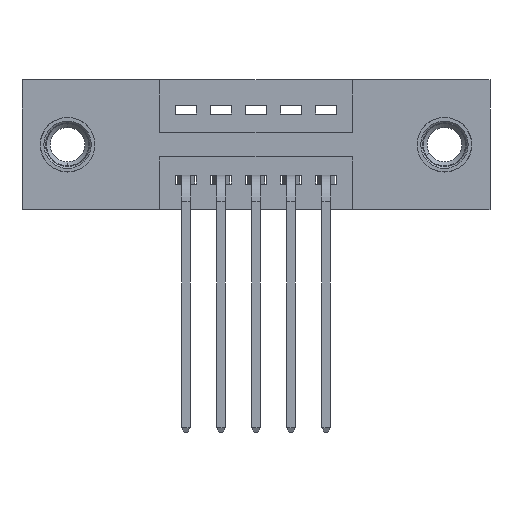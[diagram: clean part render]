
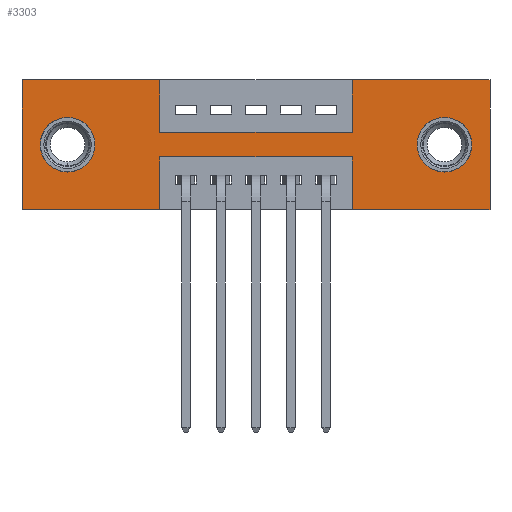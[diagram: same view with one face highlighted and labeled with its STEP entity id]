
A CAD part, front view. The second image highlights one B-rep face of the part: STEP entity #3303.
In plain terms, the highlighted planar face has unit normal (0, -1, 0).
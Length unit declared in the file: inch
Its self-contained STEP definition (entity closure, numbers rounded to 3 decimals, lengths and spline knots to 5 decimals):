
#11 = LINE ( 'NONE', #4275, #3894 ) ;
#39 = LINE ( 'NONE', #323, #8531 ) ;
#146 = CARTESIAN_POINT ( 'NONE',  ( 1.205, 0., -0.185 ) ) ;
#201 = VECTOR ( 'NONE', #7948, 39.37008 ) ;
#323 = CARTESIAN_POINT ( 'NONE',  ( 0.3925, 0., -0.37 ) ) ;
#498 = EDGE_CURVE ( 'NONE', #9425, #2298, #8544, .T. ) ;
#508 = FACE_OUTER_BOUND ( 'NONE', #5006, .T. ) ;
#535 = CARTESIAN_POINT ( 'NONE',  ( 0., 0., -0.37 ) ) ;
#790 = ORIENTED_EDGE ( 'NONE', *, *, #2302, .F. ) ;
#950 = DIRECTION ( 'NONE',  ( 0., 0., 1. ) ) ;
#1063 = DIRECTION ( 'NONE',  ( 0., 0., -1. ) ) ;
#1074 = LINE ( 'NONE', #3281, #6831 ) ;
#1170 = EDGE_CURVE ( 'NONE', #6178, #2041, #39, .T. ) ;
#1175 = DIRECTION ( 'NONE',  ( -1., 0., 0. ) ) ;
#1281 = CARTESIAN_POINT ( 'NONE',  ( 0., 0., 0. ) ) ;
#1316 = DIRECTION ( 'NONE',  ( 0., -1., 0. ) ) ;
#1618 = CARTESIAN_POINT ( 'NONE',  ( 0., 0., -0.37 ) ) ;
#1724 = LINE ( 'NONE', #1281, #5340 ) ;
#1753 = VERTEX_POINT ( 'NONE', #1618 ) ;
#1829 = CARTESIAN_POINT ( 'NONE',  ( 1.205, 0., -0.185 ) ) ;
#2041 = VERTEX_POINT ( 'NONE', #7589 ) ;
#2062 = VERTEX_POINT ( 'NONE', #4697 ) ;
#2151 = CARTESIAN_POINT ( 'NONE',  ( 0.3925, 0., -0.15 ) ) ;
#2238 = VERTEX_POINT ( 'NONE', #7132 ) ;
#2298 = VERTEX_POINT ( 'NONE', #9548 ) ;
#2302 = EDGE_CURVE ( 'NONE', #1753, #9924, #7620, .T. ) ;
#2320 = CIRCLE ( 'NONE', #3418, 0.078 ) ;
#2375 = EDGE_CURVE ( 'NONE', #4383, #6178, #11, .T. ) ;
#2426 = LINE ( 'NONE', #8313, #5318 ) ;
#2468 = DIRECTION ( 'NONE',  ( 0., 1., 0. ) ) ;
#2493 = VECTOR ( 'NONE', #6721, 39.37008 ) ;
#2654 = EDGE_CURVE ( 'NONE', #2041, #1753, #5104, .T. ) ;
#2685 = AXIS2_PLACEMENT_3D ( 'NONE', #535, #1316, #8268 ) ;
#2868 = VERTEX_POINT ( 'NONE', #4425 ) ;
#2888 = PLANE ( 'NONE',  #2685 ) ;
#2924 = CARTESIAN_POINT ( 'NONE',  ( 0.3925, 0., -0.22 ) ) ;
#3131 = ORIENTED_EDGE ( 'NONE', *, *, #7729, .T. ) ;
#3281 = CARTESIAN_POINT ( 'NONE',  ( 0.9425, 0., 0. ) ) ;
#3290 = AXIS2_PLACEMENT_3D ( 'NONE', #8690, #2468, #950 ) ;
#3303 = ADVANCED_FACE ( 'NONE', ( #4868, #9347, #508 ), #2888, .T. ) ;
#3386 = ORIENTED_EDGE ( 'NONE', *, *, #6322, .F. ) ;
#3418 = AXIS2_PLACEMENT_3D ( 'NONE', #146, #6374, #7135 ) ;
#3602 = EDGE_CURVE ( 'NONE', #8687, #8686, #4376, .T. ) ;
#3663 = CARTESIAN_POINT ( 'NONE',  ( 1.335, 0., -0.37 ) ) ;
#3681 = EDGE_CURVE ( 'NONE', #5368, #4383, #6166, .T. ) ;
#3765 = LINE ( 'NONE', #2151, #5587 ) ;
#3801 = EDGE_CURVE ( 'NONE', #9924, #2062, #1724, .T. ) ;
#3894 = VECTOR ( 'NONE', #1175, 39.37008 ) ;
#4030 = VECTOR ( 'NONE', #1063, 39.37008 ) ;
#4070 = ORIENTED_EDGE ( 'NONE', *, *, #498, .T. ) ;
#4084 = AXIS2_PLACEMENT_3D ( 'NONE', #9554, #4218, #4990 ) ;
#4094 = CARTESIAN_POINT ( 'NONE',  ( 1.335, 0., 0. ) ) ;
#4204 = VERTEX_POINT ( 'NONE', #5545 ) ;
#4218 = DIRECTION ( 'NONE',  ( 0., 1., 0. ) ) ;
#4253 = DIRECTION ( 'NONE',  ( 1., 0., 0. ) ) ;
#4275 = CARTESIAN_POINT ( 'NONE',  ( 0.3925, 0., -0.22 ) ) ;
#4323 = DIRECTION ( 'NONE',  ( -1., 0., 0. ) ) ;
#4329 = LINE ( 'NONE', #7915, #201 ) ;
#4376 = CIRCLE ( 'NONE', #8908, 0.078 ) ;
#4383 = VERTEX_POINT ( 'NONE', #6255 ) ;
#4425 = CARTESIAN_POINT ( 'NONE',  ( 1.335, 0., 0. ) ) ;
#4474 = ORIENTED_EDGE ( 'NONE', *, *, #2375, .F. ) ;
#4478 = DIRECTION ( 'NONE',  ( 0., 0., -1. ) ) ;
#4697 = CARTESIAN_POINT ( 'NONE',  ( 0.3925, 0., 0. ) ) ;
#4845 = ORIENTED_EDGE ( 'NONE', *, *, #3681, .F. ) ;
#4868 = FACE_BOUND ( 'NONE', #8288, .T. ) ;
#4982 = CARTESIAN_POINT ( 'NONE',  ( 0., 0., 0. ) ) ;
#4990 = DIRECTION ( 'NONE',  ( 0., 0., 1. ) ) ;
#5001 = DIRECTION ( 'NONE',  ( 0., 0., 1. ) ) ;
#5006 = EDGE_LOOP ( 'NONE', ( #6796, #4474, #4845, #3386, #8309, #6114, #8317, #7991, #9247, #8164, #790, #5122 ) ) ;
#5029 = CARTESIAN_POINT ( 'NONE',  ( 0., 0., -0.37 ) ) ;
#5104 = LINE ( 'NONE', #5029, #9345 ) ;
#5122 = ORIENTED_EDGE ( 'NONE', *, *, #2654, .F. ) ;
#5318 = VECTOR ( 'NONE', #4478, 39.37008 ) ;
#5340 = VECTOR ( 'NONE', #4253, 39.37008 ) ;
#5368 = VERTEX_POINT ( 'NONE', #5894 ) ;
#5423 = DIRECTION ( 'NONE',  ( 1., 0., 0. ) ) ;
#5545 = CARTESIAN_POINT ( 'NONE',  ( 0.3925, 0., -0.15 ) ) ;
#5587 = VECTOR ( 'NONE', #5423, 39.37008 ) ;
#5664 = ORIENTED_EDGE ( 'NONE', *, *, #3602, .T. ) ;
#5689 = CARTESIAN_POINT ( 'NONE',  ( 0., 0., 0. ) ) ;
#5704 = DIRECTION ( 'NONE',  ( 0., 0., -1. ) ) ;
#5797 = EDGE_LOOP ( 'NONE', ( #8000, #4070 ) ) ;
#5813 = VECTOR ( 'NONE', #5001, 39.37008 ) ;
#5894 = CARTESIAN_POINT ( 'NONE',  ( 0.9425, 0., -0.37 ) ) ;
#5900 = VERTEX_POINT ( 'NONE', #6093 ) ;
#5974 = CARTESIAN_POINT ( 'NONE',  ( 0., 0., -0.37 ) ) ;
#5996 = DIRECTION ( 'NONE',  ( 0., 0., -1. ) ) ;
#6093 = CARTESIAN_POINT ( 'NONE',  ( 0.9425, 0., 0. ) ) ;
#6114 = ORIENTED_EDGE ( 'NONE', *, *, #9998, .F. ) ;
#6166 = LINE ( 'NONE', #6626, #5813 ) ;
#6178 = VERTEX_POINT ( 'NONE', #2924 ) ;
#6255 = CARTESIAN_POINT ( 'NONE',  ( 0.9425, 0., -0.22 ) ) ;
#6303 = CIRCLE ( 'NONE', #3290, 0.078 ) ;
#6322 = EDGE_CURVE ( 'NONE', #8152, #5368, #7045, .T. ) ;
#6374 = DIRECTION ( 'NONE',  ( 0., 1., 0. ) ) ;
#6626 = CARTESIAN_POINT ( 'NONE',  ( 0.9425, 0., -0.37 ) ) ;
#6696 = CARTESIAN_POINT ( 'NONE',  ( 1.205, 0., -0.107 ) ) ;
#6721 = DIRECTION ( 'NONE',  ( -1., 0., 0. ) ) ;
#6796 = ORIENTED_EDGE ( 'NONE', *, *, #1170, .F. ) ;
#6831 = VECTOR ( 'NONE', #7843, 39.37008 ) ;
#6843 = CARTESIAN_POINT ( 'NONE',  ( 0.13, 0., -0.263 ) ) ;
#7045 = LINE ( 'NONE', #5974, #2493 ) ;
#7132 = CARTESIAN_POINT ( 'NONE',  ( 0.9425, 0., -0.15 ) ) ;
#7135 = DIRECTION ( 'NONE',  ( 0., 0., -1. ) ) ;
#7140 = EDGE_CURVE ( 'NONE', #2868, #8152, #9475, .T. ) ;
#7220 = DIRECTION ( 'NONE',  ( 0., 1., 0. ) ) ;
#7512 = EDGE_CURVE ( 'NONE', #4204, #2238, #3765, .T. ) ;
#7589 = CARTESIAN_POINT ( 'NONE',  ( 0.3925, 0., -0.37 ) ) ;
#7620 = LINE ( 'NONE', #4982, #9240 ) ;
#7657 = EDGE_CURVE ( 'NONE', #2298, #9425, #6303, .T. ) ;
#7729 = EDGE_CURVE ( 'NONE', #8686, #8687, #2320, .T. ) ;
#7843 = DIRECTION ( 'NONE',  ( 0., 0., 1. ) ) ;
#7915 = CARTESIAN_POINT ( 'NONE',  ( 0., 0., 0. ) ) ;
#7948 = DIRECTION ( 'NONE',  ( 1., 0., 0. ) ) ;
#7991 = ORIENTED_EDGE ( 'NONE', *, *, #7512, .F. ) ;
#8000 = ORIENTED_EDGE ( 'NONE', *, *, #7657, .T. ) ;
#8152 = VERTEX_POINT ( 'NONE', #3663 ) ;
#8164 = ORIENTED_EDGE ( 'NONE', *, *, #3801, .F. ) ;
#8246 = CARTESIAN_POINT ( 'NONE',  ( 1.205, 0., -0.263 ) ) ;
#8268 = DIRECTION ( 'NONE',  ( 0., 0., -1. ) ) ;
#8288 = EDGE_LOOP ( 'NONE', ( #5664, #3131 ) ) ;
#8309 = ORIENTED_EDGE ( 'NONE', *, *, #7140, .F. ) ;
#8313 = CARTESIAN_POINT ( 'NONE',  ( 0.3925, 0., 0. ) ) ;
#8317 = ORIENTED_EDGE ( 'NONE', *, *, #9807, .F. ) ;
#8531 = VECTOR ( 'NONE', #5996, 39.37008 ) ;
#8544 = CIRCLE ( 'NONE', #4084, 0.078 ) ;
#8686 = VERTEX_POINT ( 'NONE', #8246 ) ;
#8687 = VERTEX_POINT ( 'NONE', #6696 ) ;
#8690 = CARTESIAN_POINT ( 'NONE',  ( 0.13, 0., -0.185 ) ) ;
#8747 = EDGE_CURVE ( 'NONE', #2062, #4204, #2426, .T. ) ;
#8792 = DIRECTION ( 'NONE',  ( 0., 0., 1. ) ) ;
#8908 = AXIS2_PLACEMENT_3D ( 'NONE', #1829, #7220, #5704 ) ;
#9240 = VECTOR ( 'NONE', #8792, 39.37008 ) ;
#9247 = ORIENTED_EDGE ( 'NONE', *, *, #8747, .F. ) ;
#9345 = VECTOR ( 'NONE', #4323, 39.37008 ) ;
#9347 = FACE_BOUND ( 'NONE', #5797, .T. ) ;
#9425 = VERTEX_POINT ( 'NONE', #6843 ) ;
#9475 = LINE ( 'NONE', #4094, #4030 ) ;
#9548 = CARTESIAN_POINT ( 'NONE',  ( 0.13, 0., -0.107 ) ) ;
#9554 = CARTESIAN_POINT ( 'NONE',  ( 0.13, 0., -0.185 ) ) ;
#9807 = EDGE_CURVE ( 'NONE', #2238, #5900, #1074, .T. ) ;
#9924 = VERTEX_POINT ( 'NONE', #5689 ) ;
#9998 = EDGE_CURVE ( 'NONE', #5900, #2868, #4329, .T. ) ;
